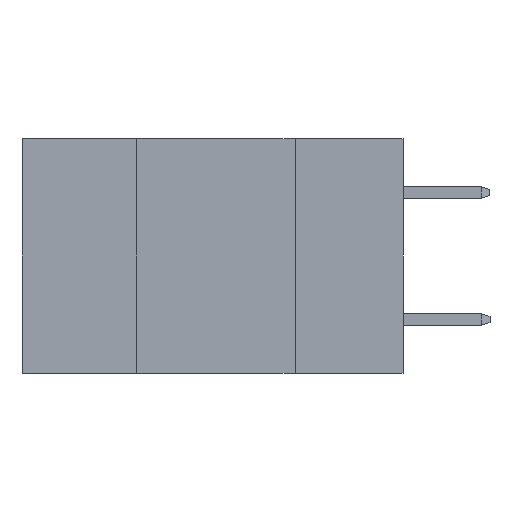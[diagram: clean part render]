
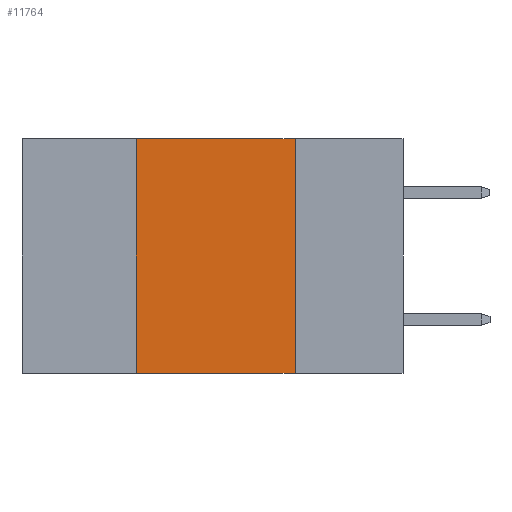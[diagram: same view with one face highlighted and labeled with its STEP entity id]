
A CAD part, left-side view. The second image highlights one B-rep face of the part: STEP entity #11764.
In plain terms, the highlighted planar face has unit normal (-1, 0, 0).
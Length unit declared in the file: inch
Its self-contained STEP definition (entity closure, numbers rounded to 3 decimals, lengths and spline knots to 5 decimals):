
#439 = LINE ( 'NONE', #581, #5567 ) ;
#581 = CARTESIAN_POINT ( 'NONE',  ( 0., 0.6, 0. ) ) ;
#665 = DIRECTION ( 'NONE',  ( 0., 0., -1. ) ) ;
#910 = VERTEX_POINT ( 'NONE', #4528 ) ;
#1191 = DIRECTION ( 'NONE',  ( 0., 0., 1. ) ) ;
#1531 = VECTOR ( 'NONE', #11309, 39.37008 ) ;
#1666 = DIRECTION ( 'NONE',  ( 0., -1., 0. ) ) ;
#1867 = DIRECTION ( 'NONE',  ( 0., 0., -1. ) ) ;
#2166 = VECTOR ( 'NONE', #665, 39.37008 ) ;
#2353 = ORIENTED_EDGE ( 'NONE', *, *, #12991, .T. ) ;
#3384 = ORIENTED_EDGE ( 'NONE', *, *, #10379, .F. ) ;
#3696 = CARTESIAN_POINT ( 'NONE',  ( 0., 0.6, -0.37 ) ) ;
#3767 = LINE ( 'NONE', #11593, #2166 ) ;
#3986 = ORIENTED_EDGE ( 'NONE', *, *, #12398, .F. ) ;
#4089 = EDGE_LOOP ( 'NONE', ( #3384, #9347, #3986, #2353 ) ) ;
#4528 = CARTESIAN_POINT ( 'NONE',  ( 0., 0.42, 0. ) ) ;
#4964 = AXIS2_PLACEMENT_3D ( 'NONE', #13075, #6479, #1867 ) ;
#5201 = CARTESIAN_POINT ( 'NONE',  ( 0., 0.42, -0.37 ) ) ;
#5567 = VECTOR ( 'NONE', #1666, 39.37008 ) ;
#6479 = DIRECTION ( 'NONE',  ( 1., 0., 0. ) ) ;
#6677 = LINE ( 'NONE', #11053, #11845 ) ;
#6683 = EDGE_CURVE ( 'NONE', #910, #6819, #439, .T. ) ;
#6803 = VERTEX_POINT ( 'NONE', #5201 ) ;
#6819 = VERTEX_POINT ( 'NONE', #10871 ) ;
#6933 = LINE ( 'NONE', #3696, #1531 ) ;
#9347 = ORIENTED_EDGE ( 'NONE', *, *, #6683, .F. ) ;
#10379 = EDGE_CURVE ( 'NONE', #6819, #12013, #3767, .T. ) ;
#10871 = CARTESIAN_POINT ( 'NONE',  ( 0., 0.17, 0. ) ) ;
#11053 = CARTESIAN_POINT ( 'NONE',  ( 0., 0.42, 0. ) ) ;
#11309 = DIRECTION ( 'NONE',  ( 0., -1., 0. ) ) ;
#11593 = CARTESIAN_POINT ( 'NONE',  ( 0., 0.17, 0. ) ) ;
#11709 = PLANE ( 'NONE',  #4964 ) ;
#11764 = ADVANCED_FACE ( 'NONE', ( #14166 ), #11709, .F. ) ;
#11845 = VECTOR ( 'NONE', #1191, 39.37008 ) ;
#12013 = VERTEX_POINT ( 'NONE', #12276 ) ;
#12276 = CARTESIAN_POINT ( 'NONE',  ( 0., 0.17, -0.37 ) ) ;
#12398 = EDGE_CURVE ( 'NONE', #6803, #910, #6677, .T. ) ;
#12991 = EDGE_CURVE ( 'NONE', #6803, #12013, #6933, .T. ) ;
#13075 = CARTESIAN_POINT ( 'NONE',  ( 0., 0.6, 0. ) ) ;
#14166 = FACE_OUTER_BOUND ( 'NONE', #4089, .T. ) ;
